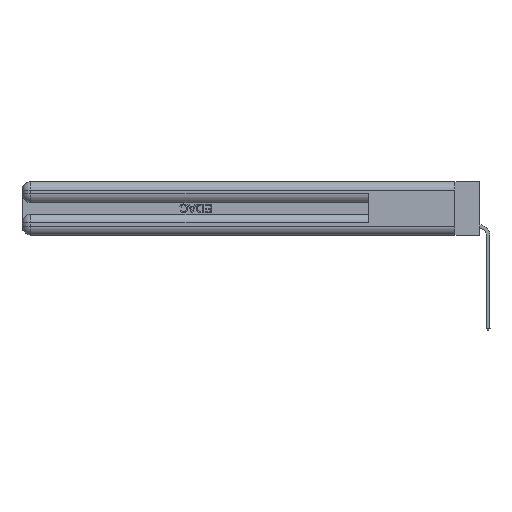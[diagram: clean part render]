
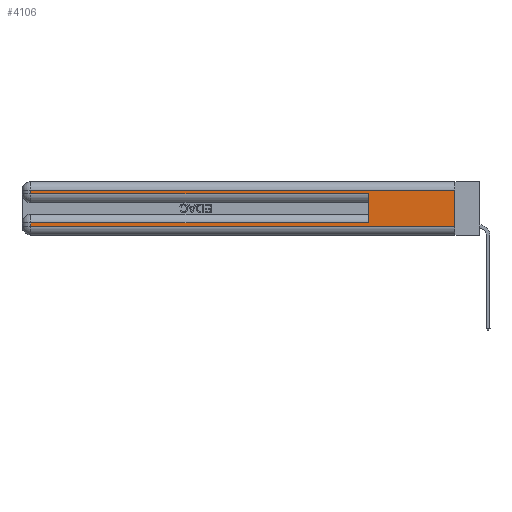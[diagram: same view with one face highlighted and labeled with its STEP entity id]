
A CAD part, left-side view. The second image highlights one B-rep face of the part: STEP entity #4106.
In plain terms, the highlighted planar face has unit normal (-1, 0, 0).
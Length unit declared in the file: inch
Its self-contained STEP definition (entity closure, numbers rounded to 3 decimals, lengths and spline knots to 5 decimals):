
#664 = DIRECTION ( 'NONE',  ( 0., 0., -1. ) ) ;
#761 = EDGE_LOOP ( 'NONE', ( #15900, #32505, #31635, #14400, #2144, #11466, #34226, #34598 ) ) ;
#1074 = CARTESIAN_POINT ( 'NONE',  ( 0., 0., 0.31 ) ) ;
#1278 = VERTEX_POINT ( 'NONE', #26452 ) ;
#1505 = VERTEX_POINT ( 'NONE', #6940 ) ;
#1759 = CARTESIAN_POINT ( 'NONE',  ( 0., 2.94, 0.085 ) ) ;
#2144 = ORIENTED_EDGE ( 'NONE', *, *, #17585, .F. ) ;
#2720 = CARTESIAN_POINT ( 'NONE',  ( 0., 2.94, 0.06 ) ) ;
#2795 = EDGE_CURVE ( 'NONE', #1278, #23341, #17480, .T. ) ;
#3652 = DIRECTION ( 'NONE',  ( 0., 1., 0. ) ) ;
#3734 = DIRECTION ( 'NONE',  ( 0., 0., -1. ) ) ;
#4106 = ADVANCED_FACE ( 'NONE', ( #33332 ), #16739, .F. ) ;
#4321 = DIRECTION ( 'NONE',  ( 0., 0., 1. ) ) ;
#4852 = LINE ( 'NONE', #32322, #31218 ) ;
#4911 = VECTOR ( 'NONE', #3652, 39.37008 ) ;
#5879 = CARTESIAN_POINT ( 'NONE',  ( 0., 2.94, 0.31 ) ) ;
#6141 = EDGE_CURVE ( 'NONE', #33415, #7762, #22208, .T. ) ;
#6313 = CARTESIAN_POINT ( 'NONE',  ( 0., 0., 0.285 ) ) ;
#6940 = CARTESIAN_POINT ( 'NONE',  ( 0., 0., 0.06 ) ) ;
#7033 = VERTEX_POINT ( 'NONE', #2720 ) ;
#7762 = VERTEX_POINT ( 'NONE', #16491 ) ;
#8125 = LINE ( 'NONE', #16138, #17810 ) ;
#8247 = LINE ( 'NONE', #13207, #21144 ) ;
#10552 = DIRECTION ( 'NONE',  ( 0., 0., -1. ) ) ;
#10651 = VECTOR ( 'NONE', #23367, 39.37008 ) ;
#11466 = ORIENTED_EDGE ( 'NONE', *, *, #2795, .T. ) ;
#13207 = CARTESIAN_POINT ( 'NONE',  ( 0., 2.94, 0.37 ) ) ;
#13719 = EDGE_CURVE ( 'NONE', #22546, #33415, #8125, .T. ) ;
#14400 = ORIENTED_EDGE ( 'NONE', *, *, #6141, .T. ) ;
#14851 = CARTESIAN_POINT ( 'NONE',  ( 0., 0., 0.31 ) ) ;
#15724 = CARTESIAN_POINT ( 'NONE',  ( 0., 0.6, 0.145 ) ) ;
#15900 = ORIENTED_EDGE ( 'NONE', *, *, #30150, .F. ) ;
#16138 = CARTESIAN_POINT ( 'NONE',  ( 0., 2.94, 0.37 ) ) ;
#16320 = DIRECTION ( 'NONE',  ( 0., 0., -1. ) ) ;
#16491 = CARTESIAN_POINT ( 'NONE',  ( 0., 0.6, 0.285 ) ) ;
#16739 = PLANE ( 'NONE',  #34612 ) ;
#17480 = LINE ( 'NONE', #31746, #10651 ) ;
#17585 = EDGE_CURVE ( 'NONE', #1278, #7762, #31973, .T. ) ;
#17810 = VECTOR ( 'NONE', #16320, 39.37008 ) ;
#18986 = EDGE_CURVE ( 'NONE', #28468, #22546, #30948, .T. ) ;
#20800 = EDGE_CURVE ( 'NONE', #7033, #1505, #4852, .T. ) ;
#21144 = VECTOR ( 'NONE', #10552, 39.37008 ) ;
#22208 = LINE ( 'NONE', #6313, #33509 ) ;
#22546 = VERTEX_POINT ( 'NONE', #5879 ) ;
#22603 = VECTOR ( 'NONE', #4321, 39.37008 ) ;
#23005 = LINE ( 'NONE', #33872, #33245 ) ;
#23341 = VERTEX_POINT ( 'NONE', #1759 ) ;
#23367 = DIRECTION ( 'NONE',  ( 0., 1., 0. ) ) ;
#26452 = CARTESIAN_POINT ( 'NONE',  ( 0., 0.6, 0.085 ) ) ;
#27127 = EDGE_CURVE ( 'NONE', #23341, #7033, #8247, .T. ) ;
#27741 = DIRECTION ( 'NONE',  ( 0., -1., 0. ) ) ;
#28162 = DIRECTION ( 'NONE',  ( 1., 0., 0. ) ) ;
#28468 = VERTEX_POINT ( 'NONE', #1074 ) ;
#30150 = EDGE_CURVE ( 'NONE', #28468, #1505, #23005, .T. ) ;
#30948 = LINE ( 'NONE', #14851, #4911 ) ;
#31218 = VECTOR ( 'NONE', #35003, 39.37008 ) ;
#31635 = ORIENTED_EDGE ( 'NONE', *, *, #13719, .T. ) ;
#31746 = CARTESIAN_POINT ( 'NONE',  ( 0., 0., 0.085 ) ) ;
#31973 = LINE ( 'NONE', #15724, #22603 ) ;
#32322 = CARTESIAN_POINT ( 'NONE',  ( 0., 0., 0.06 ) ) ;
#32505 = ORIENTED_EDGE ( 'NONE', *, *, #18986, .T. ) ;
#33245 = VECTOR ( 'NONE', #3734, 39.37008 ) ;
#33332 = FACE_OUTER_BOUND ( 'NONE', #761, .T. ) ;
#33415 = VERTEX_POINT ( 'NONE', #34715 ) ;
#33509 = VECTOR ( 'NONE', #27741, 39.37008 ) ;
#33675 = CARTESIAN_POINT ( 'NONE',  ( 0., 0., 0.37 ) ) ;
#33872 = CARTESIAN_POINT ( 'NONE',  ( 0., 0., 0.37 ) ) ;
#34226 = ORIENTED_EDGE ( 'NONE', *, *, #27127, .T. ) ;
#34598 = ORIENTED_EDGE ( 'NONE', *, *, #20800, .T. ) ;
#34612 = AXIS2_PLACEMENT_3D ( 'NONE', #33675, #28162, #664 ) ;
#34715 = CARTESIAN_POINT ( 'NONE',  ( 0., 2.94, 0.285 ) ) ;
#35003 = DIRECTION ( 'NONE',  ( 0., -1., 0. ) ) ;
